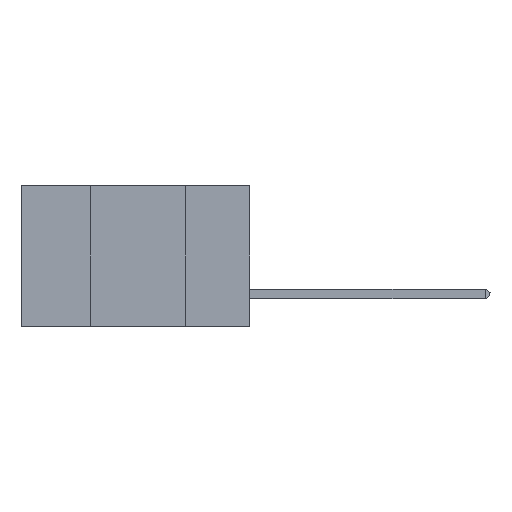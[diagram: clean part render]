
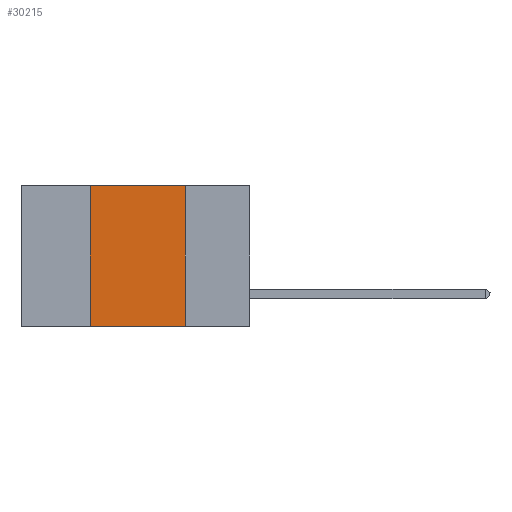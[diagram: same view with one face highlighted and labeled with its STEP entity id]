
A CAD part, left-side view. The second image highlights one B-rep face of the part: STEP entity #30215.
In plain terms, the highlighted planar face has unit normal (-1, 0, 0).
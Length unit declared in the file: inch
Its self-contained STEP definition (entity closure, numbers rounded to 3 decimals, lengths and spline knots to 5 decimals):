
#22 = AXIS2_PLACEMENT_3D ( 'NONE', #9090, #39104, #36340 ) ;
#1712 = DIRECTION ( 'NONE',  ( 0., -1., 0. ) ) ;
#6547 = VERTEX_POINT ( 'NONE', #25113 ) ;
#6612 = VECTOR ( 'NONE', #23612, 39.37008 ) ;
#7182 = VECTOR ( 'NONE', #25473, 39.37008 ) ;
#7823 = CARTESIAN_POINT ( 'NONE',  ( 0., 0.42, 0. ) ) ;
#9090 = CARTESIAN_POINT ( 'NONE',  ( 0., 0.6, 0. ) ) ;
#9225 = VECTOR ( 'NONE', #1712, 39.37008 ) ;
#9743 = EDGE_CURVE ( 'NONE', #6547, #38073, #36219, .T. ) ;
#11438 = CARTESIAN_POINT ( 'NONE',  ( 0., 0.17, 0. ) ) ;
#12950 = EDGE_CURVE ( 'NONE', #6547, #16388, #22726, .T. ) ;
#14173 = CARTESIAN_POINT ( 'NONE',  ( 0., 0.42, 0. ) ) ;
#14399 = ORIENTED_EDGE ( 'NONE', *, *, #12950, .F. ) ;
#15065 = CARTESIAN_POINT ( 'NONE',  ( 0., 0.17, -0.37 ) ) ;
#15885 = CARTESIAN_POINT ( 'NONE',  ( 0., 0.6, 0. ) ) ;
#16388 = VERTEX_POINT ( 'NONE', #7823 ) ;
#18722 = FACE_OUTER_BOUND ( 'NONE', #22410, .T. ) ;
#22052 = LINE ( 'NONE', #25916, #30995 ) ;
#22410 = EDGE_LOOP ( 'NONE', ( #30713, #34607, #14399, #23523 ) ) ;
#22726 = LINE ( 'NONE', #14173, #6612 ) ;
#23523 = ORIENTED_EDGE ( 'NONE', *, *, #9743, .T. ) ;
#23612 = DIRECTION ( 'NONE',  ( 0., 0., 1. ) ) ;
#23685 = PLANE ( 'NONE',  #22 ) ;
#25113 = CARTESIAN_POINT ( 'NONE',  ( 0., 0.42, -0.37 ) ) ;
#25473 = DIRECTION ( 'NONE',  ( 0., -1., 0. ) ) ;
#25916 = CARTESIAN_POINT ( 'NONE',  ( 0., 0.17, 0. ) ) ;
#26172 = DIRECTION ( 'NONE',  ( 0., 0., -1. ) ) ;
#29946 = VERTEX_POINT ( 'NONE', #11438 ) ;
#30215 = ADVANCED_FACE ( 'NONE', ( #18722 ), #23685, .F. ) ;
#30713 = ORIENTED_EDGE ( 'NONE', *, *, #39110, .F. ) ;
#30995 = VECTOR ( 'NONE', #26172, 39.37008 ) ;
#31271 = LINE ( 'NONE', #15885, #7182 ) ;
#32169 = CARTESIAN_POINT ( 'NONE',  ( 0., 0.6, -0.37 ) ) ;
#33316 = EDGE_CURVE ( 'NONE', #16388, #29946, #31271, .T. ) ;
#34607 = ORIENTED_EDGE ( 'NONE', *, *, #33316, .F. ) ;
#36219 = LINE ( 'NONE', #32169, #9225 ) ;
#36340 = DIRECTION ( 'NONE',  ( 0., 0., -1. ) ) ;
#38073 = VERTEX_POINT ( 'NONE', #15065 ) ;
#39104 = DIRECTION ( 'NONE',  ( 1., 0., 0. ) ) ;
#39110 = EDGE_CURVE ( 'NONE', #29946, #38073, #22052, .T. ) ;
